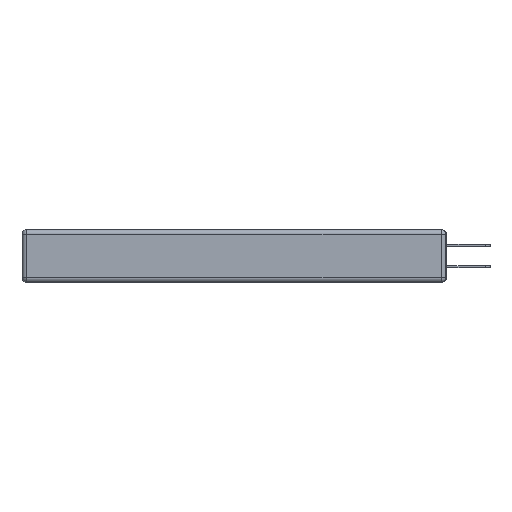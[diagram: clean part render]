
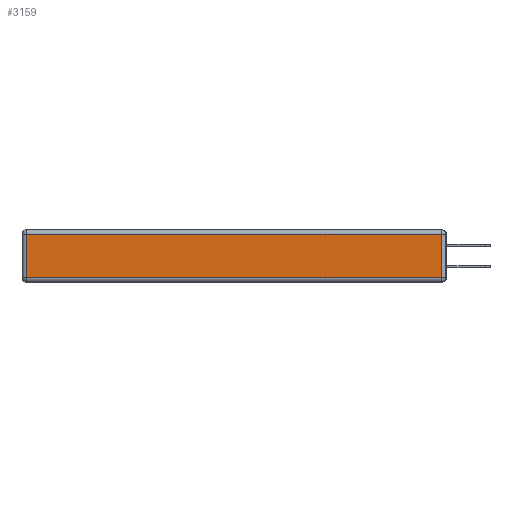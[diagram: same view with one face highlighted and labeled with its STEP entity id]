
A CAD part, left-side view. The second image highlights one B-rep face of the part: STEP entity #3159.
In plain terms, the highlighted planar face has unit normal (-1, 0, 0).
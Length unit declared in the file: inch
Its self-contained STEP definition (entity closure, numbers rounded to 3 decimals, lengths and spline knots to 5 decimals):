
#110 = CARTESIAN_POINT ( 'NONE',  ( 0., 0.03, -0.313 ) ) ;
#172 = CARTESIAN_POINT ( 'NONE',  ( 0., 0., -0.313 ) ) ;
#448 = CARTESIAN_POINT ( 'NONE',  ( 0., 2.75, -0.03 ) ) ;
#684 = CARTESIAN_POINT ( 'NONE',  ( 0., 0., -0.343 ) ) ;
#1130 = FACE_OUTER_BOUND ( 'NONE', #1140, .T. ) ;
#1140 = EDGE_LOOP ( 'NONE', ( #1898, #1678, #8463, #14993 ) ) ;
#1678 = ORIENTED_EDGE ( 'NONE', *, *, #8857, .T. ) ;
#1898 = ORIENTED_EDGE ( 'NONE', *, *, #2248, .T. ) ;
#2248 = EDGE_CURVE ( 'NONE', #7135, #6132, #11012, .T. ) ;
#2705 = DIRECTION ( 'NONE',  ( 0., 0., 1. ) ) ;
#3159 = ADVANCED_FACE ( 'NONE', ( #1130 ), #12023, .T. ) ;
#4754 = LINE ( 'NONE', #9415, #11955 ) ;
#4894 = LINE ( 'NONE', #448, #7796 ) ;
#6132 = VERTEX_POINT ( 'NONE', #110 ) ;
#6391 = EDGE_CURVE ( 'NONE', #15878, #7135, #10447, .T. ) ;
#7135 = VERTEX_POINT ( 'NONE', #9558 ) ;
#7172 = VECTOR ( 'NONE', #12998, 39.37008 ) ;
#7796 = VECTOR ( 'NONE', #10662, 39.37008 ) ;
#8463 = ORIENTED_EDGE ( 'NONE', *, *, #15431, .T. ) ;
#8483 = CARTESIAN_POINT ( 'NONE',  ( 0., 0.03, -0.03 ) ) ;
#8857 = EDGE_CURVE ( 'NONE', #6132, #14715, #4754, .T. ) ;
#9415 = CARTESIAN_POINT ( 'NONE',  ( 0., 0.03, -0.343 ) ) ;
#9558 = CARTESIAN_POINT ( 'NONE',  ( 0., 2.72, -0.313 ) ) ;
#9800 = DIRECTION ( 'NONE',  ( -1., 0., 0. ) ) ;
#10447 = LINE ( 'NONE', #15136, #11098 ) ;
#10662 = DIRECTION ( 'NONE',  ( 0., 1., 0. ) ) ;
#11012 = LINE ( 'NONE', #172, #7172 ) ;
#11098 = VECTOR ( 'NONE', #13583, 39.37008 ) ;
#11702 = CARTESIAN_POINT ( 'NONE',  ( 0., 2.72, -0.03 ) ) ;
#11955 = VECTOR ( 'NONE', #16554, 39.37008 ) ;
#12023 = PLANE ( 'NONE',  #13026 ) ;
#12998 = DIRECTION ( 'NONE',  ( 0., -1., 0. ) ) ;
#13026 = AXIS2_PLACEMENT_3D ( 'NONE', #684, #9800, #2705 ) ;
#13583 = DIRECTION ( 'NONE',  ( 0., 0., -1. ) ) ;
#14715 = VERTEX_POINT ( 'NONE', #8483 ) ;
#14993 = ORIENTED_EDGE ( 'NONE', *, *, #6391, .T. ) ;
#15136 = CARTESIAN_POINT ( 'NONE',  ( 0., 2.72, -0.343 ) ) ;
#15431 = EDGE_CURVE ( 'NONE', #14715, #15878, #4894, .T. ) ;
#15878 = VERTEX_POINT ( 'NONE', #11702 ) ;
#16554 = DIRECTION ( 'NONE',  ( 0., 0., 1. ) ) ;
